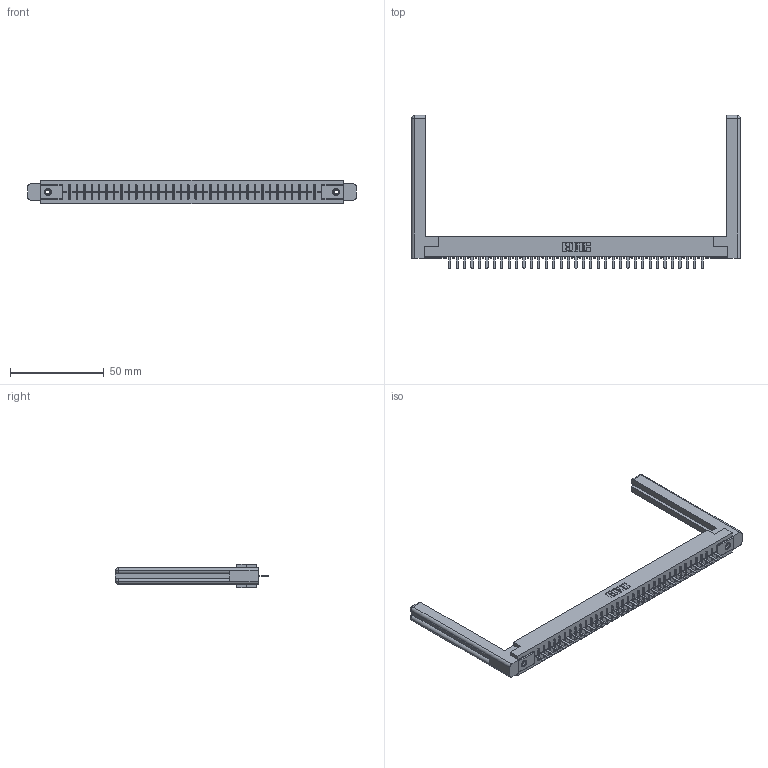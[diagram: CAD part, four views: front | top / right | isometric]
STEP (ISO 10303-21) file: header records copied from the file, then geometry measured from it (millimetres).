
FILE_DESCRIPTION (( 'STEP AP203' ), '1' );
FILE_NAME ('356-035-520-158.STEP', '2018-08-01T21:44:37', ( '' ), ( '' ), 'SwSTEP 2.0', 'SolidWorks 2016', '' );
FILE_SCHEMA (( 'CONFIG_CONTROL_DESIGN' ));
Length unit declared in the file: inch
Products named in the file (5): 306 Part_.156 Dia; 306-290-001_120; 345-250-001_345-250-001-102; 307-220-058; 356-035-520-158
Assembly tree (40 placements, depth 2):
  356-035-520-158
    306 Part_.156 Dia
    306-290-001_120  x35
    345-250-001_345-250-001-102  x2
    307-220-058  x2
Bounding box: 175.31 x 81.76 x 12.7 mm (x, y, z)
Volume: 26398.6 mm3; surface area: 24903.6 mm2
Topology: 40 solids, 40 shells, 2708 faces, 7565 edges, 4842 vertices
Faces by surface type: plane 1797, cylinder 747, sphere 140, cone 12, torus 12
Entity records: 36135 total; most frequent: CARTESIAN_POINT 6075, ORIENTED_EDGE 5964, DIRECTION 5946, EDGE_CURVE 2982, LINE 2324, VECTOR 2324, VERTEX_POINT 1886, AXIS2_PLACEMENT_3D 1811
